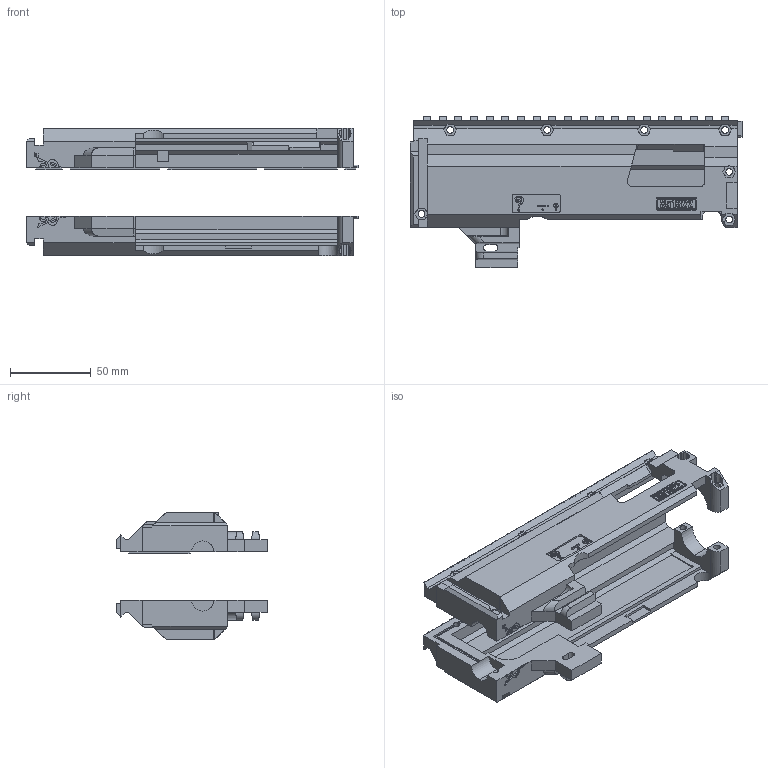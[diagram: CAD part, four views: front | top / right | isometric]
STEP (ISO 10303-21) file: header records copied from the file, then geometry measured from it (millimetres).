
FILE_DESCRIPTION(('STEP AP214'),'1');
FILE_NAME('Are we czech yet Upper receiver w_ bolt holes lip clearance.stp','2020-10-09T16:47:22',(' '),(' '),'Spatial InterOp 3D',' ',' ');
FILE_SCHEMA(('AUTOMOTIVE_DESIGN { 1 0 10303 214 1 1 1 1 }'));
Length unit declared in the file: metre
Products named in the file (5): Are We CZech Yet UPPER RECEIVER 351322 v8 mod; Left; Right; Are We CZech Yet UPPER RECEIVER Chonky; Are we czech yet Upper receiver w_ bolt holes lip clearance
Assembly tree (4 placements, depth 4):
  Are we czech yet Upper receiver w_ bolt holes lip clearance
    Are We CZech Yet UPPER RECEIVER Chonky
      Are We CZech Yet UPPER RECEIVER 351322 v8 mod
        Left
        Right
Bounding box: 206 x 93.96 x 78.89 mm (x, y, z)
Volume: 234049.7 mm3; surface area: 89181.1 mm2
Topology: 2 solids, 2 shells, 1590 faces, 4584 edges, 3053 vertices
Faces by surface type: plane 1243, cylinder 265, extrusion 72, bspline 6, torus 4
Entity records: 54410 total; most frequent: CARTESIAN_POINT 12163, ORIENTED_EDGE 9168, DIRECTION 8104, EDGE_CURVE 4584, VECTOR 3950, LINE 3878, VERTEX_POINT 3053, AXIS2_PLACEMENT_3D 2077
